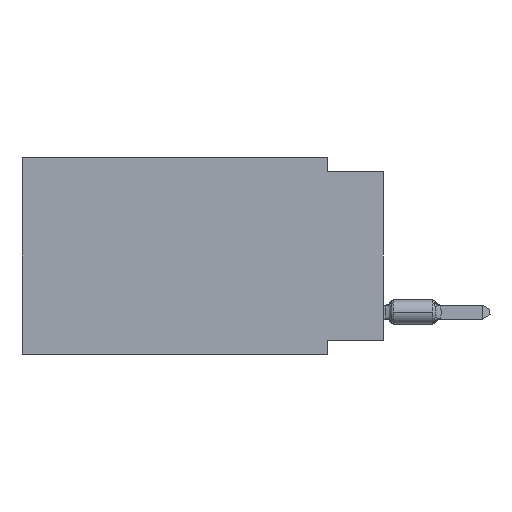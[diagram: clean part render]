
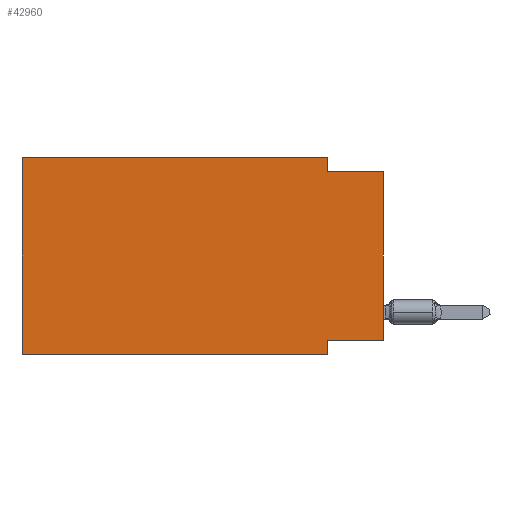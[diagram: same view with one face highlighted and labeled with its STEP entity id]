
A CAD part, left-side view. The second image highlights one B-rep face of the part: STEP entity #42960.
In plain terms, the highlighted planar face has unit normal (-1, 0, 0).
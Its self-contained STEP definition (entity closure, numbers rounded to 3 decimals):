
#1317 = EDGE_CURVE ( 'NONE', #20528, #55390, #1953, .T. ) ;
#1953 = LINE ( 'NONE', #6577, #11902 ) ;
#4623 = VERTEX_POINT ( 'NONE', #56220 ) ;
#4924 = DIRECTION ( 'NONE',  ( 0., -1., 0. ) ) ;
#5391 = DIRECTION ( 'NONE',  ( 0., 1., 0. ) ) ;
#5550 = ORIENTED_EDGE ( 'NONE', *, *, #1317, .F. ) ;
#6152 = EDGE_CURVE ( 'NONE', #43616, #54213, #8158, .T. ) ;
#6577 = CARTESIAN_POINT ( 'NONE',  ( 0., 16.383, 0. ) ) ;
#8158 = LINE ( 'NONE', #26708, #50191 ) ;
#8505 = VERTEX_POINT ( 'NONE', #56247 ) ;
#8915 = ORIENTED_EDGE ( 'NONE', *, *, #13947, .T. ) ;
#9711 = VECTOR ( 'NONE', #54485, 1000. ) ;
#10572 = DIRECTION ( 'NONE',  ( 1., 0., 0. ) ) ;
#11902 = VECTOR ( 'NONE', #24272, 1000. ) ;
#12959 = VECTOR ( 'NONE', #14071, 1000. ) ;
#13373 = DIRECTION ( 'NONE',  ( 0., 0., -1. ) ) ;
#13947 = EDGE_CURVE ( 'NONE', #8505, #4623, #24279, .T. ) ;
#14071 = DIRECTION ( 'NONE',  ( 0., -1., 0. ) ) ;
#14260 = EDGE_CURVE ( 'NONE', #18422, #4623, #35780, .T. ) ;
#14652 = CARTESIAN_POINT ( 'NONE',  ( 0., 16.383, 0. ) ) ;
#16166 = EDGE_CURVE ( 'NONE', #21306, #18422, #28749, .T. ) ;
#17547 = ORIENTED_EDGE ( 'NONE', *, *, #6152, .F. ) ;
#18422 = VERTEX_POINT ( 'NONE', #48656 ) ;
#19157 = AXIS2_PLACEMENT_3D ( 'NONE', #14652, #10572, #27992 ) ;
#20528 = VERTEX_POINT ( 'NONE', #27391 ) ;
#20844 = DIRECTION ( 'NONE',  ( 0., -1., 0. ) ) ;
#21306 = VERTEX_POINT ( 'NONE', #54039 ) ;
#22525 = LINE ( 'NONE', #40727, #49065 ) ;
#23933 = FACE_OUTER_BOUND ( 'NONE', #43282, .T. ) ;
#24272 = DIRECTION ( 'NONE',  ( 0., 0., 1. ) ) ;
#24279 = LINE ( 'NONE', #50852, #43448 ) ;
#24843 = ORIENTED_EDGE ( 'NONE', *, *, #16166, .F. ) ;
#25206 = LINE ( 'NONE', #42845, #38165 ) ;
#26708 = CARTESIAN_POINT ( 'NONE',  ( 0., 2.54, -8.89 ) ) ;
#27391 = CARTESIAN_POINT ( 'NONE',  ( 0., 16.383, -8.89 ) ) ;
#27992 = DIRECTION ( 'NONE',  ( 0., 0., -1. ) ) ;
#28614 = EDGE_CURVE ( 'NONE', #55390, #21306, #25206, .T. ) ;
#28749 = LINE ( 'NONE', #36849, #9711 ) ;
#29752 = CARTESIAN_POINT ( 'NONE',  ( 0., 2.54, -8.89 ) ) ;
#31273 = CARTESIAN_POINT ( 'NONE',  ( 0., 16.383, -8.89 ) ) ;
#32241 = EDGE_CURVE ( 'NONE', #20528, #54213, #44868, .T. ) ;
#32823 = VECTOR ( 'NONE', #4924, 1000. ) ;
#35505 = CARTESIAN_POINT ( 'NONE',  ( 0., 0., -0.635 ) ) ;
#35780 = LINE ( 'NONE', #35505, #12959 ) ;
#36089 = PLANE ( 'NONE',  #19157 ) ;
#36849 = CARTESIAN_POINT ( 'NONE',  ( 0., 2.54, 0. ) ) ;
#38165 = VECTOR ( 'NONE', #20844, 1000. ) ;
#38717 = CARTESIAN_POINT ( 'NONE',  ( 0., 16.383, 0. ) ) ;
#40727 = CARTESIAN_POINT ( 'NONE',  ( 0., 0., -8.255 ) ) ;
#41895 = EDGE_CURVE ( 'NONE', #8505, #43616, #22525, .T. ) ;
#42845 = CARTESIAN_POINT ( 'NONE',  ( 0., 16.383, 0. ) ) ;
#42960 = ADVANCED_FACE ( 'NONE', ( #23933 ), #36089, .F. ) ;
#43039 = ORIENTED_EDGE ( 'NONE', *, *, #41895, .F. ) ;
#43282 = EDGE_LOOP ( 'NONE', ( #8915, #48534, #24843, #45088, #5550, #49413, #17547, #43039 ) ) ;
#43448 = VECTOR ( 'NONE', #50283, 1000. ) ;
#43503 = CARTESIAN_POINT ( 'NONE',  ( 0., 2.54, -8.255 ) ) ;
#43616 = VERTEX_POINT ( 'NONE', #43503 ) ;
#44868 = LINE ( 'NONE', #31273, #32823 ) ;
#45088 = ORIENTED_EDGE ( 'NONE', *, *, #28614, .F. ) ;
#48534 = ORIENTED_EDGE ( 'NONE', *, *, #14260, .F. ) ;
#48656 = CARTESIAN_POINT ( 'NONE',  ( 0., 2.54, -0.635 ) ) ;
#49065 = VECTOR ( 'NONE', #5391, 1000. ) ;
#49413 = ORIENTED_EDGE ( 'NONE', *, *, #32241, .T. ) ;
#50191 = VECTOR ( 'NONE', #13373, 1000. ) ;
#50283 = DIRECTION ( 'NONE',  ( 0., 0., 1. ) ) ;
#50852 = CARTESIAN_POINT ( 'NONE',  ( 0., 0., 0. ) ) ;
#54039 = CARTESIAN_POINT ( 'NONE',  ( 0., 2.54, 0. ) ) ;
#54213 = VERTEX_POINT ( 'NONE', #29752 ) ;
#54485 = DIRECTION ( 'NONE',  ( 0., 0., -1. ) ) ;
#55390 = VERTEX_POINT ( 'NONE', #38717 ) ;
#56220 = CARTESIAN_POINT ( 'NONE',  ( 0., 0., -0.635 ) ) ;
#56247 = CARTESIAN_POINT ( 'NONE',  ( 0., 0., -8.255 ) ) ;
